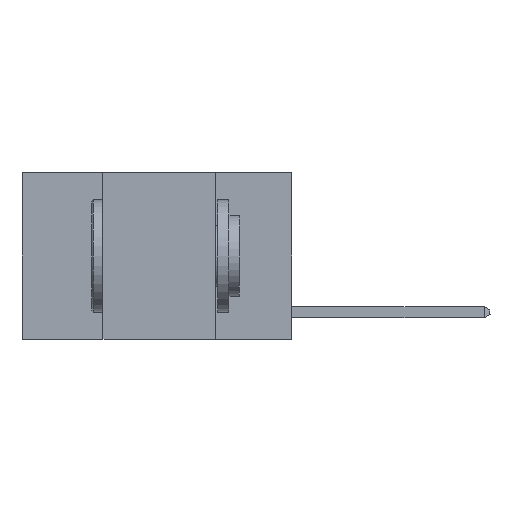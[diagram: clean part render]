
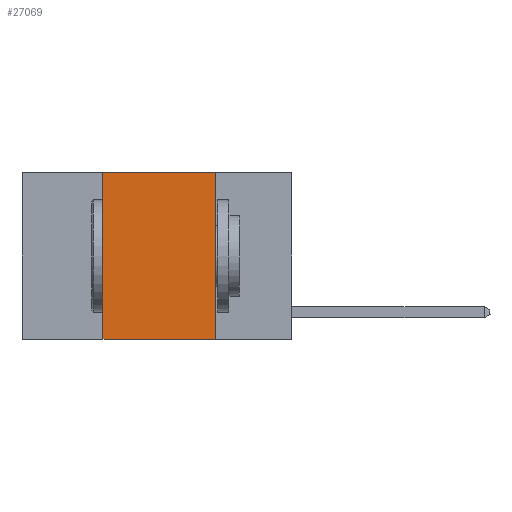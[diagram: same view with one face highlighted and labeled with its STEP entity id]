
A CAD part, left-side view. The second image highlights one B-rep face of the part: STEP entity #27069.
In plain terms, the highlighted planar face has unit normal (-1, 0, 0).
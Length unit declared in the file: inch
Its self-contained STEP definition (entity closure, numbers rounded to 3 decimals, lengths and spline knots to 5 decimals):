
#579 = VERTEX_POINT ( 'NONE', #4546 ) ;
#684 = AXIS2_PLACEMENT_3D ( 'NONE', #24031, #22140, #26530 ) ;
#770 = EDGE_CURVE ( 'NONE', #10107, #17436, #16612, .T. ) ;
#3491 = EDGE_LOOP ( 'NONE', ( #19546, #24318, #20462, #11065 ) ) ;
#4546 = CARTESIAN_POINT ( 'NONE',  ( 0., 0.42, 0. ) ) ;
#5025 = CARTESIAN_POINT ( 'NONE',  ( 0., 0.6, 0. ) ) ;
#6711 = FACE_OUTER_BOUND ( 'NONE', #3491, .T. ) ;
#8689 = CARTESIAN_POINT ( 'NONE',  ( 0., 0.17, -0.37 ) ) ;
#8881 = VECTOR ( 'NONE', #13434, 39.37008 ) ;
#10107 = VERTEX_POINT ( 'NONE', #23471 ) ;
#10261 = VECTOR ( 'NONE', #24385, 39.37008 ) ;
#11065 = ORIENTED_EDGE ( 'NONE', *, *, #24907, .T. ) ;
#11304 = EDGE_CURVE ( 'NONE', #579, #10107, #13901, .T. ) ;
#13434 = DIRECTION ( 'NONE',  ( 0., 0., 1. ) ) ;
#13901 = LINE ( 'NONE', #5025, #24617 ) ;
#15504 = CARTESIAN_POINT ( 'NONE',  ( 0., 0.6, -0.37 ) ) ;
#16031 = DIRECTION ( 'NONE',  ( 0., 0., -1. ) ) ;
#16612 = LINE ( 'NONE', #25483, #26459 ) ;
#17436 = VERTEX_POINT ( 'NONE', #8689 ) ;
#17724 = LINE ( 'NONE', #15504, #10261 ) ;
#19546 = ORIENTED_EDGE ( 'NONE', *, *, #770, .F. ) ;
#19694 = LINE ( 'NONE', #19829, #8881 ) ;
#19829 = CARTESIAN_POINT ( 'NONE',  ( 0., 0.42, 0. ) ) ;
#20462 = ORIENTED_EDGE ( 'NONE', *, *, #23751, .F. ) ;
#21696 = PLANE ( 'NONE',  #684 ) ;
#22140 = DIRECTION ( 'NONE',  ( 1., 0., 0. ) ) ;
#22778 = DIRECTION ( 'NONE',  ( 0., -1., 0. ) ) ;
#23309 = CARTESIAN_POINT ( 'NONE',  ( 0., 0.42, -0.37 ) ) ;
#23471 = CARTESIAN_POINT ( 'NONE',  ( 0., 0.17, 0. ) ) ;
#23751 = EDGE_CURVE ( 'NONE', #23977, #579, #19694, .T. ) ;
#23977 = VERTEX_POINT ( 'NONE', #23309 ) ;
#24031 = CARTESIAN_POINT ( 'NONE',  ( 0., 0.6, 0. ) ) ;
#24318 = ORIENTED_EDGE ( 'NONE', *, *, #11304, .F. ) ;
#24385 = DIRECTION ( 'NONE',  ( 0., -1., 0. ) ) ;
#24617 = VECTOR ( 'NONE', #22778, 39.37008 ) ;
#24907 = EDGE_CURVE ( 'NONE', #23977, #17436, #17724, .T. ) ;
#25483 = CARTESIAN_POINT ( 'NONE',  ( 0., 0.17, 0. ) ) ;
#26459 = VECTOR ( 'NONE', #16031, 39.37008 ) ;
#26530 = DIRECTION ( 'NONE',  ( 0., 0., -1. ) ) ;
#27069 = ADVANCED_FACE ( 'NONE', ( #6711 ), #21696, .F. ) ;
